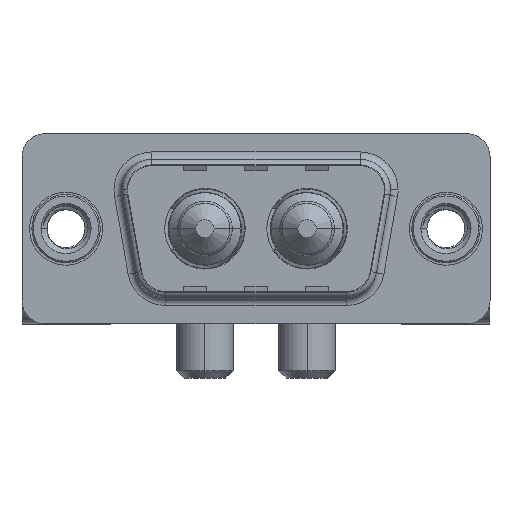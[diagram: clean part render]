
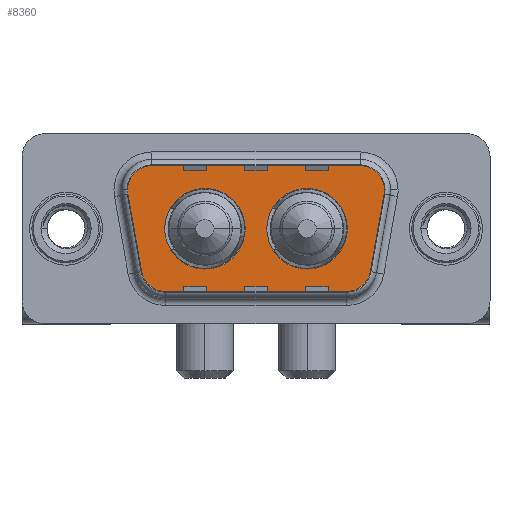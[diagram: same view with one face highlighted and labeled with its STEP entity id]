
A CAD part, top view. The second image highlights one B-rep face of the part: STEP entity #8360.
In plain terms, the highlighted planar face has unit normal (0, 0, 1).
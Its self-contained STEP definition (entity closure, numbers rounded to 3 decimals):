
#183 = VERTEX_POINT ( 'NONE', #10155 ) ;
#241 = EDGE_LOOP ( 'NONE', ( #12312, #585 ) ) ;
#318 = CARTESIAN_POINT ( 'NONE',  ( 6.49, 0., 0. ) ) ;
#389 = EDGE_CURVE ( 'NONE', #7160, #5893, #11583, .T. ) ;
#546 = DIRECTION ( 'NONE',  ( -1., 0., 0. ) ) ;
#582 = CARTESIAN_POINT ( 'NONE',  ( 9.14, 0., 0. ) ) ;
#585 = ORIENTED_EDGE ( 'NONE', *, *, #1174, .F. ) ;
#613 = FACE_BOUND ( 'NONE', #1322, .T. ) ;
#719 = CARTESIAN_POINT ( 'NONE',  ( 6.459, -4.9, 0. ) ) ;
#741 = ORIENTED_EDGE ( 'NONE', *, *, #12418, .T. ) ;
#1073 = CIRCLE ( 'NONE', #6023, 2. ) ;
#1174 = EDGE_CURVE ( 'NONE', #12364, #7667, #1888, .T. ) ;
#1177 = VECTOR ( 'NONE', #10115, 1000. ) ;
#1206 = DIRECTION ( 'NONE',  ( 0., 0., 1. ) ) ;
#1322 = EDGE_LOOP ( 'NONE', ( #11748, #10587 ) ) ;
#1395 = CARTESIAN_POINT ( 'NONE',  ( 3.466, 2.553, 0. ) ) ;
#1524 = EDGE_LOOP ( 'NONE', ( #7513, #8703, #10484, #11477, #741, #12191, #7091, #13431, #5844 ) ) ;
#1769 = EDGE_CURVE ( 'NONE', #5893, #13264, #7073, .T. ) ;
#1888 = CIRCLE ( 'NONE', #2336, 2.65 ) ;
#1891 = CIRCLE ( 'NONE', #12299, 2.65 ) ;
#2336 = AXIS2_PLACEMENT_3D ( 'NONE', #582, #7955, #9026 ) ;
#2470 = EDGE_CURVE ( 'NONE', #7803, #7815, #6774, .T. ) ;
#2481 = VECTOR ( 'NONE', #7920, 1000. ) ;
#2643 = VECTOR ( 'NONE', #8359, 1000. ) ;
#2726 = EDGE_CURVE ( 'NONE', #7263, #3789, #12012, .T. ) ;
#2825 = CIRCLE ( 'NONE', #6216, 2. ) ;
#3245 = EDGE_CURVE ( 'NONE', #7815, #13179, #2825, .T. ) ;
#3250 = CARTESIAN_POINT ( 'NONE',  ( 18.541, -4.9, 0. ) ) ;
#3355 = CARTESIAN_POINT ( 'NONE',  ( 5.436, 4.9, 0. ) ) ;
#3418 = VERTEX_POINT ( 'NONE', #3612 ) ;
#3612 = CARTESIAN_POINT ( 'NONE',  ( 21.564, 2.9, 0. ) ) ;
#3789 = VERTEX_POINT ( 'NONE', #9767 ) ;
#3815 = CARTESIAN_POINT ( 'NONE',  ( 19.564, 4.9, 0. ) ) ;
#3860 = DIRECTION ( 'NONE',  ( 1., 0., 0. ) ) ;
#3950 = CARTESIAN_POINT ( 'NONE',  ( 18.541, -2.9, 0. ) ) ;
#4206 = CARTESIAN_POINT ( 'NONE',  ( 15.86, 0., 0. ) ) ;
#4367 = CARTESIAN_POINT ( 'NONE',  ( 11.79, 0., 0. ) ) ;
#4431 = AXIS2_PLACEMENT_3D ( 'NONE', #9756, #8623, #4499 ) ;
#4489 = LINE ( 'NONE', #3355, #1177 ) ;
#4499 = DIRECTION ( 'NONE',  ( 1., 0., 0. ) ) ;
#4557 = CARTESIAN_POINT ( 'NONE',  ( 9.14, 0., 0. ) ) ;
#4638 = AXIS2_PLACEMENT_3D ( 'NONE', #4206, #12751, #13972 ) ;
#4773 = FACE_BOUND ( 'NONE', #241, .T. ) ;
#4874 = DIRECTION ( 'NONE',  ( 0., 0., 1. ) ) ;
#4924 = CARTESIAN_POINT ( 'NONE',  ( 18.541, -2.9, 0. ) ) ;
#4932 = CARTESIAN_POINT ( 'NONE',  ( 21.534, 2.553, 0. ) ) ;
#5070 = DIRECTION ( 'NONE',  ( 0., 0., 1. ) ) ;
#5439 = DIRECTION ( 'NONE',  ( 0., 0., 1. ) ) ;
#5499 = AXIS2_PLACEMENT_3D ( 'NONE', #4924, #13483, #3860 ) ;
#5844 = ORIENTED_EDGE ( 'NONE', *, *, #11222, .T. ) ;
#5893 = VERTEX_POINT ( 'NONE', #10722 ) ;
#5940 = EDGE_CURVE ( 'NONE', #3789, #7263, #1891, .T. ) ;
#6004 = DIRECTION ( 'NONE',  ( 0.174, 0.985, 0. ) ) ;
#6023 = AXIS2_PLACEMENT_3D ( 'NONE', #12634, #5070, #546 ) ;
#6064 = DIRECTION ( 'NONE',  ( 1., 0., 0. ) ) ;
#6146 = LINE ( 'NONE', #10628, #2643 ) ;
#6216 = AXIS2_PLACEMENT_3D ( 'NONE', #10857, #13157, #8874 ) ;
#6643 = AXIS2_PLACEMENT_3D ( 'NONE', #4557, #8910, #6064 ) ;
#6774 = LINE ( 'NONE', #1395, #2481 ) ;
#7073 = LINE ( 'NONE', #4932, #13938 ) ;
#7091 = ORIENTED_EDGE ( 'NONE', *, *, #2470, .T. ) ;
#7160 = VERTEX_POINT ( 'NONE', #3250 ) ;
#7203 = EDGE_CURVE ( 'NONE', #13264, #3418, #12993, .T. ) ;
#7210 = FACE_OUTER_BOUND ( 'NONE', #1524, .T. ) ;
#7263 = VERTEX_POINT ( 'NONE', #8868 ) ;
#7454 = DIRECTION ( 'NONE',  ( -1., 0., 0. ) ) ;
#7513 = ORIENTED_EDGE ( 'NONE', *, *, #389, .T. ) ;
#7667 = VERTEX_POINT ( 'NONE', #4367 ) ;
#7803 = VERTEX_POINT ( 'NONE', #7995 ) ;
#7815 = VERTEX_POINT ( 'NONE', #8853 ) ;
#7920 = DIRECTION ( 'NONE',  ( 0.174, -0.985, 0. ) ) ;
#7955 = DIRECTION ( 'NONE',  ( 0., 0., 1. ) ) ;
#7995 = CARTESIAN_POINT ( 'NONE',  ( 3.466, 2.553, 0. ) ) ;
#8015 = CIRCLE ( 'NONE', #6643, 2.65 ) ;
#8236 = EDGE_CURVE ( 'NONE', #7667, #12364, #8015, .T. ) ;
#8359 = DIRECTION ( 'NONE',  ( 1., 0., 0. ) ) ;
#8360 = ADVANCED_FACE ( 'NONE', ( #613, #4773, #7210 ), #9116, .T. ) ;
#8623 = DIRECTION ( 'NONE',  ( 0., 0., 1. ) ) ;
#8703 = ORIENTED_EDGE ( 'NONE', *, *, #1769, .T. ) ;
#8853 = CARTESIAN_POINT ( 'NONE',  ( 4.489, -3.247, 0. ) ) ;
#8868 = CARTESIAN_POINT ( 'NONE',  ( 13.21, 0., 0. ) ) ;
#8871 = DIRECTION ( 'NONE',  ( 1., 0., 0. ) ) ;
#8874 = DIRECTION ( 'NONE',  ( -1., 0., 0. ) ) ;
#8910 = DIRECTION ( 'NONE',  ( 0., 0., 1. ) ) ;
#9026 = DIRECTION ( 'NONE',  ( 1., 0., 0. ) ) ;
#9071 = AXIS2_PLACEMENT_3D ( 'NONE', #3950, #4874, #13580 ) ;
#9116 = PLANE ( 'NONE',  #5499 ) ;
#9756 = CARTESIAN_POINT ( 'NONE',  ( 5.436, 2.9, 0. ) ) ;
#9767 = CARTESIAN_POINT ( 'NONE',  ( 18.51, 0., 0. ) ) ;
#10115 = DIRECTION ( 'NONE',  ( -1., 0., 0. ) ) ;
#10155 = CARTESIAN_POINT ( 'NONE',  ( 5.436, 4.9, 0. ) ) ;
#10484 = ORIENTED_EDGE ( 'NONE', *, *, #7203, .T. ) ;
#10587 = ORIENTED_EDGE ( 'NONE', *, *, #2726, .F. ) ;
#10628 = CARTESIAN_POINT ( 'NONE',  ( 6.459, -4.9, 0. ) ) ;
#10722 = CARTESIAN_POINT ( 'NONE',  ( 20.511, -3.247, 0. ) ) ;
#10852 = CARTESIAN_POINT ( 'NONE',  ( 19.564, 2.9, 0. ) ) ;
#10857 = CARTESIAN_POINT ( 'NONE',  ( 6.459, -2.9, 0. ) ) ;
#11048 = VERTEX_POINT ( 'NONE', #3815 ) ;
#11142 = CARTESIAN_POINT ( 'NONE',  ( 15.86, 0., 0. ) ) ;
#11222 = EDGE_CURVE ( 'NONE', #13179, #7160, #6146, .T. ) ;
#11290 = EDGE_CURVE ( 'NONE', #183, #7803, #13558, .T. ) ;
#11415 = AXIS2_PLACEMENT_3D ( 'NONE', #10852, #1206, #7454 ) ;
#11477 = ORIENTED_EDGE ( 'NONE', *, *, #12060, .T. ) ;
#11568 = CARTESIAN_POINT ( 'NONE',  ( 21.534, 2.553, 0. ) ) ;
#11583 = CIRCLE ( 'NONE', #9071, 2. ) ;
#11748 = ORIENTED_EDGE ( 'NONE', *, *, #5940, .F. ) ;
#12012 = CIRCLE ( 'NONE', #4638, 2.65 ) ;
#12060 = EDGE_CURVE ( 'NONE', #3418, #11048, #1073, .T. ) ;
#12191 = ORIENTED_EDGE ( 'NONE', *, *, #11290, .T. ) ;
#12299 = AXIS2_PLACEMENT_3D ( 'NONE', #11142, #5439, #8871 ) ;
#12312 = ORIENTED_EDGE ( 'NONE', *, *, #8236, .F. ) ;
#12364 = VERTEX_POINT ( 'NONE', #318 ) ;
#12418 = EDGE_CURVE ( 'NONE', #11048, #183, #4489, .T. ) ;
#12634 = CARTESIAN_POINT ( 'NONE',  ( 19.564, 2.9, 0. ) ) ;
#12751 = DIRECTION ( 'NONE',  ( 0., 0., 1. ) ) ;
#12993 = CIRCLE ( 'NONE', #11415, 2. ) ;
#13157 = DIRECTION ( 'NONE',  ( 0., 0., 1. ) ) ;
#13179 = VERTEX_POINT ( 'NONE', #719 ) ;
#13264 = VERTEX_POINT ( 'NONE', #11568 ) ;
#13431 = ORIENTED_EDGE ( 'NONE', *, *, #3245, .T. ) ;
#13483 = DIRECTION ( 'NONE',  ( 0., 0., 1. ) ) ;
#13558 = CIRCLE ( 'NONE', #4431, 2. ) ;
#13580 = DIRECTION ( 'NONE',  ( 1., 0., 0. ) ) ;
#13938 = VECTOR ( 'NONE', #6004, 1000. ) ;
#13972 = DIRECTION ( 'NONE',  ( 1., 0., 0. ) ) ;
